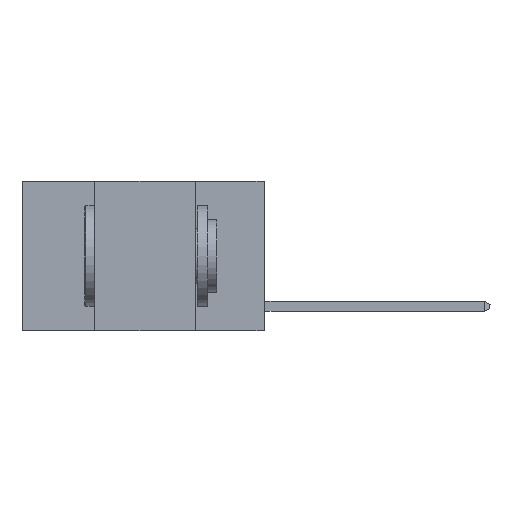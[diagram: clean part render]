
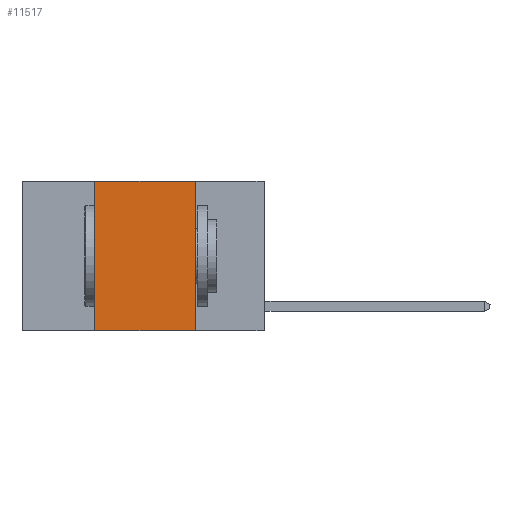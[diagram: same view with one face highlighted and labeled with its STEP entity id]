
A CAD part, left-side view. The second image highlights one B-rep face of the part: STEP entity #11517.
In plain terms, the highlighted planar face has unit normal (-1, 0, 0).
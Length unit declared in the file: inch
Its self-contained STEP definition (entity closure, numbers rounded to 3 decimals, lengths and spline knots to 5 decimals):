
#211 = CARTESIAN_POINT ( 'NONE',  ( 0., 0.17, -0.37 ) ) ;
#242 = DIRECTION ( 'NONE',  ( 1., 0., 0. ) ) ;
#489 = VERTEX_POINT ( 'NONE', #15206 ) ;
#691 = EDGE_CURVE ( 'NONE', #489, #13504, #3664, .T. ) ;
#730 = CARTESIAN_POINT ( 'NONE',  ( 0., 0.6, -0.37 ) ) ;
#808 = DIRECTION ( 'NONE',  ( 0., -1., 0. ) ) ;
#1736 = DIRECTION ( 'NONE',  ( 0., 0., -1. ) ) ;
#1983 = CARTESIAN_POINT ( 'NONE',  ( 0., 0.6, 0. ) ) ;
#2610 = FACE_OUTER_BOUND ( 'NONE', #9842, .T. ) ;
#2751 = EDGE_CURVE ( 'NONE', #11368, #13504, #8643, .T. ) ;
#3522 = LINE ( 'NONE', #12343, #15589 ) ;
#3664 = LINE ( 'NONE', #4607, #9656 ) ;
#4098 = AXIS2_PLACEMENT_3D ( 'NONE', #7533, #242, #8695 ) ;
#4607 = CARTESIAN_POINT ( 'NONE',  ( 0., 0.17, 0. ) ) ;
#5131 = PLANE ( 'NONE',  #4098 ) ;
#5642 = ORIENTED_EDGE ( 'NONE', *, *, #2751, .T. ) ;
#6006 = LINE ( 'NONE', #1983, #12375 ) ;
#6366 = DIRECTION ( 'NONE',  ( 0., 0., 1. ) ) ;
#7533 = CARTESIAN_POINT ( 'NONE',  ( 0., 0.6, 0. ) ) ;
#8046 = ORIENTED_EDGE ( 'NONE', *, *, #691, .F. ) ;
#8643 = LINE ( 'NONE', #730, #11465 ) ;
#8695 = DIRECTION ( 'NONE',  ( 0., 0., -1. ) ) ;
#9656 = VECTOR ( 'NONE', #1736, 39.37008 ) ;
#9842 = EDGE_LOOP ( 'NONE', ( #8046, #12013, #11606, #5642 ) ) ;
#11368 = VERTEX_POINT ( 'NONE', #13264 ) ;
#11465 = VECTOR ( 'NONE', #808, 39.37008 ) ;
#11517 = ADVANCED_FACE ( 'NONE', ( #2610 ), #5131, .F. ) ;
#11606 = ORIENTED_EDGE ( 'NONE', *, *, #12899, .F. ) ;
#12013 = ORIENTED_EDGE ( 'NONE', *, *, #12504, .F. ) ;
#12343 = CARTESIAN_POINT ( 'NONE',  ( 0., 0.42, 0. ) ) ;
#12375 = VECTOR ( 'NONE', #13978, 39.37008 ) ;
#12504 = EDGE_CURVE ( 'NONE', #15555, #489, #6006, .T. ) ;
#12899 = EDGE_CURVE ( 'NONE', #11368, #15555, #3522, .T. ) ;
#13264 = CARTESIAN_POINT ( 'NONE',  ( 0., 0.42, -0.37 ) ) ;
#13504 = VERTEX_POINT ( 'NONE', #211 ) ;
#13978 = DIRECTION ( 'NONE',  ( 0., -1., 0. ) ) ;
#14139 = CARTESIAN_POINT ( 'NONE',  ( 0., 0.42, 0. ) ) ;
#15206 = CARTESIAN_POINT ( 'NONE',  ( 0., 0.17, 0. ) ) ;
#15555 = VERTEX_POINT ( 'NONE', #14139 ) ;
#15589 = VECTOR ( 'NONE', #6366, 39.37008 ) ;
